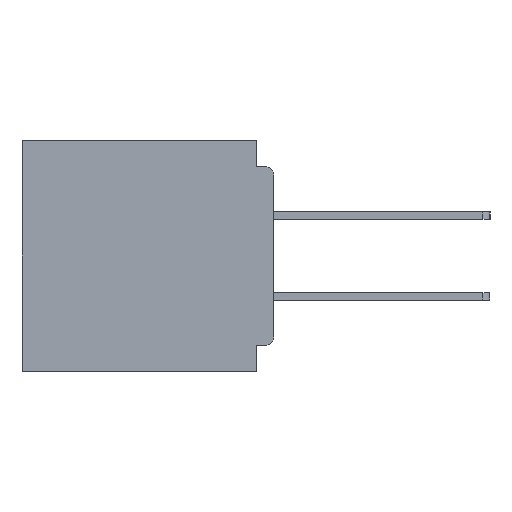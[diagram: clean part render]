
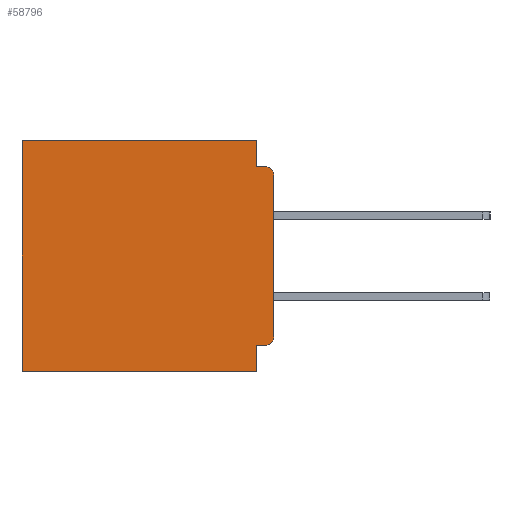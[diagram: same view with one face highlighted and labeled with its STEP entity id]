
A CAD part, left-side view. The second image highlights one B-rep face of the part: STEP entity #58796.
In plain terms, the highlighted planar face has unit normal (-1, 0, 0).
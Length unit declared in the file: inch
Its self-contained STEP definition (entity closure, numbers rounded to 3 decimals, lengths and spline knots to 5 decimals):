
#726 = VERTEX_POINT ( 'NONE', #16088 ) ;
#944 = CARTESIAN_POINT ( 'NONE',  ( 0.3, 0., -0.4 ) ) ;
#1672 = ORIENTED_EDGE ( 'NONE', *, *, #17671, .F. ) ;
#2612 = AXIS2_PLACEMENT_3D ( 'NONE', #944, #44385, #15571 ) ;
#2960 = VECTOR ( 'NONE', #58966, 39.37008 ) ;
#4224 = CARTESIAN_POINT ( 'NONE',  ( 0.3, 0.031, 0. ) ) ;
#4415 = CARTESIAN_POINT ( 'NONE',  ( 0.3, 0., -0.4 ) ) ;
#4534 = CARTESIAN_POINT ( 'NONE',  ( 0.3, 0., -0.355 ) ) ;
#4594 = VERTEX_POINT ( 'NONE', #25885 ) ;
#5797 = PLANE ( 'NONE',  #2612 ) ;
#6693 = ORIENTED_EDGE ( 'NONE', *, *, #48852, .T. ) ;
#6740 = ORIENTED_EDGE ( 'NONE', *, *, #56926, .F. ) ;
#6998 = DIRECTION ( 'NONE',  ( 0., -1., 0. ) ) ;
#8317 = AXIS2_PLACEMENT_3D ( 'NONE', #17178, #50817, #22027 ) ;
#8601 = EDGE_CURVE ( 'NONE', #55281, #55649, #27233, .T. ) ;
#10723 = DIRECTION ( 'NONE',  ( 0., 1., 0. ) ) ;
#10876 = VERTEX_POINT ( 'NONE', #59461 ) ;
#11224 = CARTESIAN_POINT ( 'NONE',  ( 0.3, 0.031, -0.4 ) ) ;
#12069 = VECTOR ( 'NONE', #6998, 39.37008 ) ;
#12980 = LINE ( 'NONE', #54072, #32618 ) ;
#13396 = FACE_OUTER_BOUND ( 'NONE', #20266, .T. ) ;
#14516 = DIRECTION ( 'NONE',  ( 0., 1., 0. ) ) ;
#14844 = CIRCLE ( 'NONE', #8317, 0.015 ) ;
#15571 = DIRECTION ( 'NONE',  ( 0., 0., -1. ) ) ;
#16088 = CARTESIAN_POINT ( 'NONE',  ( 0.3, 0., -0.06 ) ) ;
#16099 = VECTOR ( 'NONE', #16191, 39.37008 ) ;
#16191 = DIRECTION ( 'NONE',  ( 0., 0., -1. ) ) ;
#16257 = VERTEX_POINT ( 'NONE', #11224 ) ;
#17178 = CARTESIAN_POINT ( 'NONE',  ( 0.3, 0.015, -0.06 ) ) ;
#17401 = ORIENTED_EDGE ( 'NONE', *, *, #38588, .T. ) ;
#17671 = EDGE_CURVE ( 'NONE', #21775, #16257, #32586, .T. ) ;
#17814 = VECTOR ( 'NONE', #21146, 39.37008 ) ;
#17983 = DIRECTION ( 'NONE',  ( -1., 0., 0. ) ) ;
#19713 = VECTOR ( 'NONE', #41757, 39.37008 ) ;
#19888 = EDGE_CURVE ( 'NONE', #16257, #4594, #46512, .T. ) ;
#20106 = CARTESIAN_POINT ( 'NONE',  ( 0.3, 0.015, -0.045 ) ) ;
#20266 = EDGE_LOOP ( 'NONE', ( #53954, #17401, #6740, #45181, #54609, #6693, #51900, #1672, #46537, #23292 ) ) ;
#20332 = CIRCLE ( 'NONE', #27706, 0.015 ) ;
#20537 = EDGE_CURVE ( 'NONE', #21054, #21775, #44149, .T. ) ;
#21054 = VERTEX_POINT ( 'NONE', #33485 ) ;
#21146 = DIRECTION ( 'NONE',  ( 0., 0., -1. ) ) ;
#21775 = VERTEX_POINT ( 'NONE', #57916 ) ;
#22027 = DIRECTION ( 'NONE',  ( 0., 0., -1. ) ) ;
#23011 = VERTEX_POINT ( 'NONE', #20106 ) ;
#23292 = ORIENTED_EDGE ( 'NONE', *, *, #46199, .T. ) ;
#25885 = CARTESIAN_POINT ( 'NONE',  ( 0.3, 0.437, -0.4 ) ) ;
#27233 = LINE ( 'NONE', #35069, #2960 ) ;
#27284 = CARTESIAN_POINT ( 'NONE',  ( 0.3, 0.031, -0.4 ) ) ;
#27706 = AXIS2_PLACEMENT_3D ( 'NONE', #46777, #17983, #51620 ) ;
#28559 = EDGE_CURVE ( 'NONE', #726, #10876, #41707, .T. ) ;
#29930 = VECTOR ( 'NONE', #14516, 39.37008 ) ;
#30677 = LINE ( 'NONE', #54557, #17814 ) ;
#31129 = CARTESIAN_POINT ( 'NONE',  ( 0.3, 0., -0.045 ) ) ;
#31343 = VERTEX_POINT ( 'NONE', #36278 ) ;
#32586 = LINE ( 'NONE', #27284, #19713 ) ;
#32618 = VECTOR ( 'NONE', #10723, 39.37008 ) ;
#33485 = CARTESIAN_POINT ( 'NONE',  ( 0.3, 0.015, -0.355 ) ) ;
#35069 = CARTESIAN_POINT ( 'NONE',  ( 0.3, 0.031, 0. ) ) ;
#36278 = CARTESIAN_POINT ( 'NONE',  ( 0.3, 0.437, 0. ) ) ;
#38588 = EDGE_CURVE ( 'NONE', #726, #23011, #14844, .T. ) ;
#40718 = LINE ( 'NONE', #31129, #12069 ) ;
#41707 = LINE ( 'NONE', #44986, #16099 ) ;
#41757 = DIRECTION ( 'NONE',  ( 0., 0., -1. ) ) ;
#44149 = LINE ( 'NONE', #4534, #29930 ) ;
#44385 = DIRECTION ( 'NONE',  ( 1., 0., 0. ) ) ;
#44986 = CARTESIAN_POINT ( 'NONE',  ( 0.3, 0., -0.4 ) ) ;
#44993 = VECTOR ( 'NONE', #57511, 39.37008 ) ;
#45181 = ORIENTED_EDGE ( 'NONE', *, *, #8601, .F. ) ;
#45507 = CARTESIAN_POINT ( 'NONE',  ( 0.3, 0.031, -0.045 ) ) ;
#46199 = EDGE_CURVE ( 'NONE', #21054, #10876, #20332, .T. ) ;
#46512 = LINE ( 'NONE', #4415, #44993 ) ;
#46537 = ORIENTED_EDGE ( 'NONE', *, *, #20537, .F. ) ;
#46777 = CARTESIAN_POINT ( 'NONE',  ( 0.3, 0.015, -0.34 ) ) ;
#48852 = EDGE_CURVE ( 'NONE', #31343, #4594, #30677, .T. ) ;
#50817 = DIRECTION ( 'NONE',  ( -1., 0., 0. ) ) ;
#51273 = EDGE_CURVE ( 'NONE', #55281, #31343, #12980, .T. ) ;
#51620 = DIRECTION ( 'NONE',  ( 0., 0., -1. ) ) ;
#51900 = ORIENTED_EDGE ( 'NONE', *, *, #19888, .F. ) ;
#53954 = ORIENTED_EDGE ( 'NONE', *, *, #28559, .F. ) ;
#54072 = CARTESIAN_POINT ( 'NONE',  ( 0.3, 0., 0. ) ) ;
#54557 = CARTESIAN_POINT ( 'NONE',  ( 0.3, 0.437, -0.4 ) ) ;
#54609 = ORIENTED_EDGE ( 'NONE', *, *, #51273, .T. ) ;
#55281 = VERTEX_POINT ( 'NONE', #4224 ) ;
#55649 = VERTEX_POINT ( 'NONE', #45507 ) ;
#56926 = EDGE_CURVE ( 'NONE', #55649, #23011, #40718, .T. ) ;
#57511 = DIRECTION ( 'NONE',  ( 0., 1., 0. ) ) ;
#57916 = CARTESIAN_POINT ( 'NONE',  ( 0.3, 0.031, -0.355 ) ) ;
#58796 = ADVANCED_FACE ( 'NONE', ( #13396 ), #5797, .F. ) ;
#58966 = DIRECTION ( 'NONE',  ( 0., 0., -1. ) ) ;
#59461 = CARTESIAN_POINT ( 'NONE',  ( 0.3, 0., -0.34 ) ) ;
